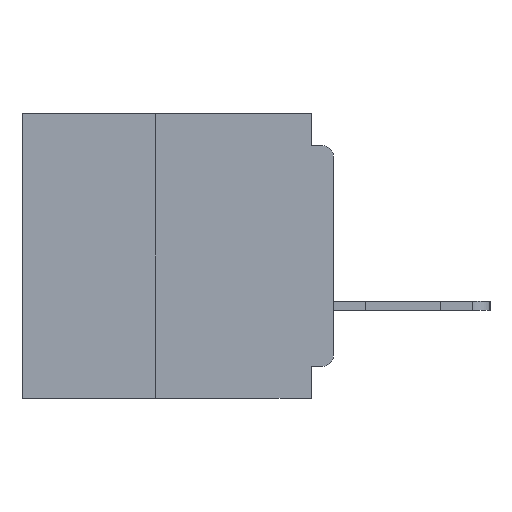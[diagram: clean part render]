
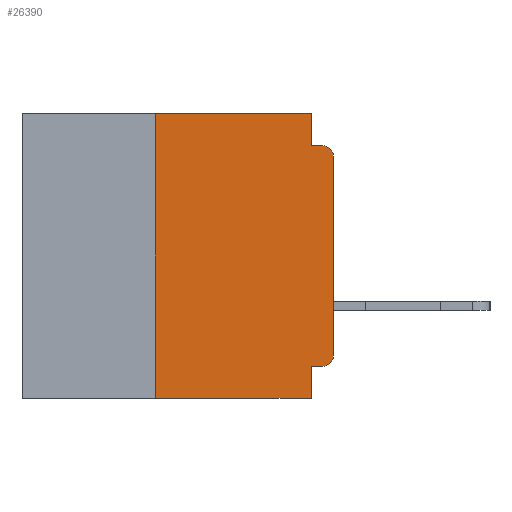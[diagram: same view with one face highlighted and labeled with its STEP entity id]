
A CAD part, left-side view. The second image highlights one B-rep face of the part: STEP entity #26390.
In plain terms, the highlighted planar face has unit normal (-1, 0, 0).
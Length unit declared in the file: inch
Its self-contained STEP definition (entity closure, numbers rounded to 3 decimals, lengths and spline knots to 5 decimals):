
#1366 = CARTESIAN_POINT ( 'NONE',  ( 0., 0.031, -0.4 ) ) ;
#2011 = AXIS2_PLACEMENT_3D ( 'NONE', #28197, #3715, #32270 ) ;
#2385 = EDGE_CURVE ( 'NONE', #44119, #24773, #16763, .T. ) ;
#2400 = ORIENTED_EDGE ( 'NONE', *, *, #20418, .T. ) ;
#2512 = VECTOR ( 'NONE', #45336, 39.37008 ) ;
#2669 = DIRECTION ( 'NONE',  ( 0., 0., -1. ) ) ;
#3020 = VERTEX_POINT ( 'NONE', #35646 ) ;
#3715 = DIRECTION ( 'NONE',  ( 1., 0., 0. ) ) ;
#3975 = EDGE_CURVE ( 'NONE', #10677, #21770, #21662, .T. ) ;
#4441 = ORIENTED_EDGE ( 'NONE', *, *, #24292, .T. ) ;
#4606 = ORIENTED_EDGE ( 'NONE', *, *, #5044, .F. ) ;
#5044 = EDGE_CURVE ( 'NONE', #3020, #21770, #43785, .T. ) ;
#5485 = CIRCLE ( 'NONE', #19832, 0.015 ) ;
#6453 = DIRECTION ( 'NONE',  ( 0., 1., 0. ) ) ;
#6702 = CARTESIAN_POINT ( 'NONE',  ( 0., 0.437, 0. ) ) ;
#6736 = VECTOR ( 'NONE', #32058, 39.37008 ) ;
#7642 = PLANE ( 'NONE',  #2011 ) ;
#9267 = VERTEX_POINT ( 'NONE', #33516 ) ;
#9346 = VERTEX_POINT ( 'NONE', #1366 ) ;
#10455 = DIRECTION ( 'NONE',  ( 0., -1., 0. ) ) ;
#10630 = CARTESIAN_POINT ( 'NONE',  ( 0., 0., -0.045 ) ) ;
#10677 = VERTEX_POINT ( 'NONE', #45783 ) ;
#13043 = DIRECTION ( 'NONE',  ( 0., 0., 1. ) ) ;
#14678 = CARTESIAN_POINT ( 'NONE',  ( 0., 0., -0.355 ) ) ;
#16319 = LINE ( 'NONE', #52364, #6736 ) ;
#16320 = LINE ( 'NONE', #26177, #48745 ) ;
#16763 = LINE ( 'NONE', #14678, #47906 ) ;
#17190 = DIRECTION ( 'NONE',  ( -1., 0., 0. ) ) ;
#18862 = DIRECTION ( 'NONE',  ( 0., -1., 0. ) ) ;
#18971 = EDGE_LOOP ( 'NONE', ( #4441, #27921, #4606, #39390, #34587, #34420, #2400, #36604, #33586, #29773 ) ) ;
#19414 = CARTESIAN_POINT ( 'NONE',  ( 0., 0., -0.34 ) ) ;
#19832 = AXIS2_PLACEMENT_3D ( 'NONE', #51412, #27160, #2669 ) ;
#20063 = CARTESIAN_POINT ( 'NONE',  ( 0., 0.015, -0.355 ) ) ;
#20418 = EDGE_CURVE ( 'NONE', #25622, #9346, #48769, .T. ) ;
#21662 = CIRCLE ( 'NONE', #36375, 0.015 ) ;
#21770 = VERTEX_POINT ( 'NONE', #32712 ) ;
#24230 = LINE ( 'NONE', #41247, #2512 ) ;
#24292 = EDGE_CURVE ( 'NONE', #40359, #10677, #36990, .T. ) ;
#24773 = VERTEX_POINT ( 'NONE', #34210 ) ;
#25622 = VERTEX_POINT ( 'NONE', #39578 ) ;
#26177 = CARTESIAN_POINT ( 'NONE',  ( 0., 0.031, 0. ) ) ;
#26390 = ADVANCED_FACE ( 'NONE', ( #28994 ), #7642, .F. ) ;
#27160 = DIRECTION ( 'NONE',  ( -1., 0., 0. ) ) ;
#27485 = VECTOR ( 'NONE', #13043, 39.37008 ) ;
#27921 = ORIENTED_EDGE ( 'NONE', *, *, #3975, .T. ) ;
#28197 = CARTESIAN_POINT ( 'NONE',  ( 0., 0.437, 0. ) ) ;
#28994 = FACE_OUTER_BOUND ( 'NONE', #18971, .T. ) ;
#29773 = ORIENTED_EDGE ( 'NONE', *, *, #49634, .T. ) ;
#30299 = DIRECTION ( 'NONE',  ( 0., 0., -1. ) ) ;
#31441 = EDGE_CURVE ( 'NONE', #46912, #3020, #16320, .T. ) ;
#31560 = CARTESIAN_POINT ( 'NONE',  ( 0., 0.437, -0.4 ) ) ;
#31756 = VECTOR ( 'NONE', #10455, 39.37008 ) ;
#32058 = DIRECTION ( 'NONE',  ( 0., 0., 1. ) ) ;
#32270 = DIRECTION ( 'NONE',  ( 0., 0., -1. ) ) ;
#32712 = CARTESIAN_POINT ( 'NONE',  ( 0., 0.015, -0.045 ) ) ;
#33516 = CARTESIAN_POINT ( 'NONE',  ( 0., 0.25, 0. ) ) ;
#33586 = ORIENTED_EDGE ( 'NONE', *, *, #2385, .F. ) ;
#34210 = CARTESIAN_POINT ( 'NONE',  ( 0., 0.031, -0.355 ) ) ;
#34420 = ORIENTED_EDGE ( 'NONE', *, *, #45452, .F. ) ;
#34542 = EDGE_CURVE ( 'NONE', #24773, #9346, #24230, .T. ) ;
#34587 = ORIENTED_EDGE ( 'NONE', *, *, #34833, .F. ) ;
#34833 = EDGE_CURVE ( 'NONE', #9267, #46912, #52109, .T. ) ;
#35646 = CARTESIAN_POINT ( 'NONE',  ( 0., 0.031, -0.045 ) ) ;
#36375 = AXIS2_PLACEMENT_3D ( 'NONE', #41520, #17190, #45618 ) ;
#36604 = ORIENTED_EDGE ( 'NONE', *, *, #34542, .F. ) ;
#36990 = LINE ( 'NONE', #49624, #27485 ) ;
#37977 = VECTOR ( 'NONE', #52055, 39.37008 ) ;
#38278 = CARTESIAN_POINT ( 'NONE',  ( 0., 0.031, 0. ) ) ;
#39390 = ORIENTED_EDGE ( 'NONE', *, *, #31441, .F. ) ;
#39578 = CARTESIAN_POINT ( 'NONE',  ( 0., 0.25, -0.4 ) ) ;
#40359 = VERTEX_POINT ( 'NONE', #19414 ) ;
#41247 = CARTESIAN_POINT ( 'NONE',  ( 0., 0.031, -0.4 ) ) ;
#41520 = CARTESIAN_POINT ( 'NONE',  ( 0., 0.015, -0.06 ) ) ;
#43785 = LINE ( 'NONE', #10630, #31756 ) ;
#44119 = VERTEX_POINT ( 'NONE', #20063 ) ;
#45336 = DIRECTION ( 'NONE',  ( 0., 0., -1. ) ) ;
#45452 = EDGE_CURVE ( 'NONE', #25622, #9267, #16319, .T. ) ;
#45618 = DIRECTION ( 'NONE',  ( 0., 0., -1. ) ) ;
#45783 = CARTESIAN_POINT ( 'NONE',  ( 0., 0., -0.06 ) ) ;
#46912 = VERTEX_POINT ( 'NONE', #38278 ) ;
#47906 = VECTOR ( 'NONE', #6453, 39.37008 ) ;
#48745 = VECTOR ( 'NONE', #30299, 39.37008 ) ;
#48769 = LINE ( 'NONE', #31560, #37977 ) ;
#49624 = CARTESIAN_POINT ( 'NONE',  ( 0., 0., 0. ) ) ;
#49634 = EDGE_CURVE ( 'NONE', #44119, #40359, #5485, .T. ) ;
#50865 = VECTOR ( 'NONE', #18862, 39.37008 ) ;
#51412 = CARTESIAN_POINT ( 'NONE',  ( 0., 0.015, -0.34 ) ) ;
#52055 = DIRECTION ( 'NONE',  ( 0., -1., 0. ) ) ;
#52109 = LINE ( 'NONE', #6702, #50865 ) ;
#52364 = CARTESIAN_POINT ( 'NONE',  ( 0., 0.25, -0.4 ) ) ;
